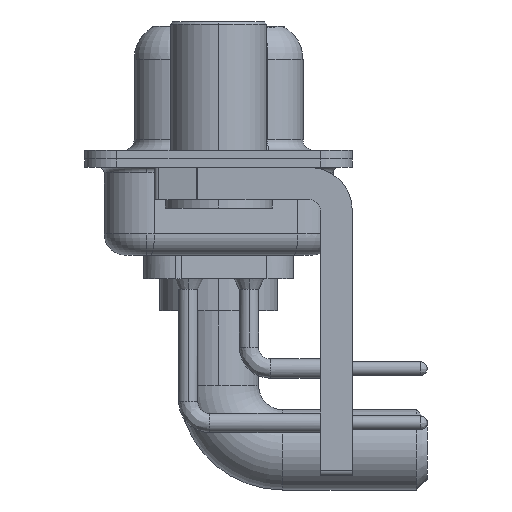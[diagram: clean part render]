
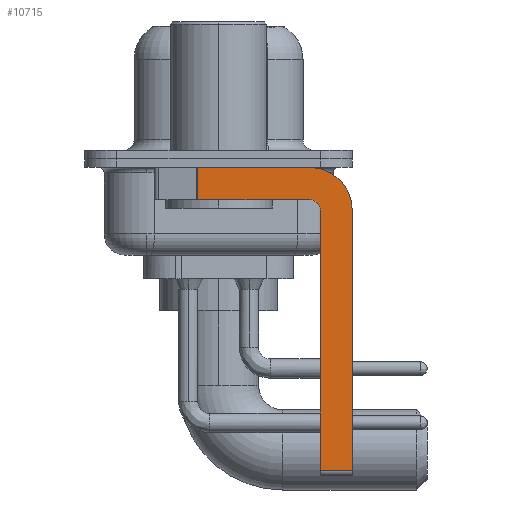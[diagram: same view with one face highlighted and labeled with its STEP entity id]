
A CAD part, left-side view. The second image highlights one B-rep face of the part: STEP entity #10715.
In plain terms, the highlighted planar face has unit normal (-1, 0, 0).
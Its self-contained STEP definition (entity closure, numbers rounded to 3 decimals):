
#270 = CARTESIAN_POINT ( 'NONE',  ( -2.9, 0.978, -1.9 ) ) ;
#313 = VECTOR ( 'NONE', #9322, 1000. ) ;
#455 = CARTESIAN_POINT ( 'NONE',  ( -2.9, -4.25, -1.9 ) ) ;
#612 = LINE ( 'NONE', #16915, #10787 ) ;
#702 = DIRECTION ( 'NONE',  ( 0., 0., -1. ) ) ;
#1063 = EDGE_CURVE ( 'NONE', #9135, #16388, #6700, .T. ) ;
#1362 = DIRECTION ( 'NONE',  ( -1., 0., 0. ) ) ;
#2097 = DIRECTION ( 'NONE',  ( 1., 0., 0. ) ) ;
#2965 = DIRECTION ( 'NONE',  ( 0., -1., 0. ) ) ;
#3438 = VERTEX_POINT ( 'NONE', #8987 ) ;
#4019 = VECTOR ( 'NONE', #702, 1000. ) ;
#4088 = VECTOR ( 'NONE', #7142, 1000. ) ;
#4329 = VECTOR ( 'NONE', #2965, 1000. ) ;
#4563 = DIRECTION ( 'NONE',  ( 0., 0., 1. ) ) ;
#4607 = CARTESIAN_POINT ( 'NONE',  ( -2.9, -4.75, -2.4 ) ) ;
#4699 = ORIENTED_EDGE ( 'NONE', *, *, #1063, .F. ) ;
#4745 = CIRCLE ( 'NONE', #13836, 0.5 ) ;
#5616 = PLANE ( 'NONE',  #11859 ) ;
#5619 = EDGE_CURVE ( 'NONE', #18272, #20762, #14762, .T. ) ;
#6700 = LINE ( 'NONE', #13361, #4088 ) ;
#7142 = DIRECTION ( 'NONE',  ( 0., 0., -1. ) ) ;
#7213 = FACE_OUTER_BOUND ( 'NONE', #13570, .T. ) ;
#7489 = DIRECTION ( 'NONE',  ( 0., -1., 0. ) ) ;
#7623 = CARTESIAN_POINT ( 'NONE',  ( -2.9, -4.25, -0.4 ) ) ;
#8331 = ORIENTED_EDGE ( 'NONE', *, *, #15761, .F. ) ;
#8383 = ORIENTED_EDGE ( 'NONE', *, *, #9776, .F. ) ;
#8558 = DIRECTION ( 'NONE',  ( 0., 0., -1. ) ) ;
#8987 = CARTESIAN_POINT ( 'NONE',  ( -2.9, -4.75, -14.55 ) ) ;
#9135 = VERTEX_POINT ( 'NONE', #17491 ) ;
#9322 = DIRECTION ( 'NONE',  ( 0., 0., 1. ) ) ;
#9467 = CIRCLE ( 'NONE', #19290, 2. ) ;
#9637 = EDGE_CURVE ( 'NONE', #14297, #12432, #4745, .T. ) ;
#9776 = EDGE_CURVE ( 'NONE', #14078, #9135, #9467, .T. ) ;
#10487 = CARTESIAN_POINT ( 'NONE',  ( -2.9, -4.25, -2.4 ) ) ;
#10715 = ADVANCED_FACE ( 'NONE', ( #7213 ), #5616, .F. ) ;
#10787 = VECTOR ( 'NONE', #19797, 1000. ) ;
#11312 = CARTESIAN_POINT ( 'NONE',  ( -2.9, -4.25, -14.55 ) ) ;
#11504 = LINE ( 'NONE', #19682, #313 ) ;
#11859 = AXIS2_PLACEMENT_3D ( 'NONE', #10487, #16946, #20717 ) ;
#12332 = LINE ( 'NONE', #18829, #18881 ) ;
#12432 = VERTEX_POINT ( 'NONE', #455 ) ;
#12444 = CARTESIAN_POINT ( 'NONE',  ( -2.9, 0.978, -1.9 ) ) ;
#13361 = CARTESIAN_POINT ( 'NONE',  ( -2.9, -6.25, -2.4 ) ) ;
#13570 = EDGE_LOOP ( 'NONE', ( #8331, #13980, #20934, #14658, #15207, #16603, #4699, #8383 ) ) ;
#13836 = AXIS2_PLACEMENT_3D ( 'NONE', #19074, #1362, #4563 ) ;
#13980 = ORIENTED_EDGE ( 'NONE', *, *, #5619, .T. ) ;
#14078 = VERTEX_POINT ( 'NONE', #7623 ) ;
#14297 = VERTEX_POINT ( 'NONE', #4607 ) ;
#14592 = LINE ( 'NONE', #11312, #4329 ) ;
#14658 = ORIENTED_EDGE ( 'NONE', *, *, #9637, .F. ) ;
#14762 = LINE ( 'NONE', #270, #4019 ) ;
#15207 = ORIENTED_EDGE ( 'NONE', *, *, #18730, .F. ) ;
#15461 = EDGE_CURVE ( 'NONE', #3438, #16388, #14592, .T. ) ;
#15761 = EDGE_CURVE ( 'NONE', #18272, #14078, #12332, .T. ) ;
#16388 = VERTEX_POINT ( 'NONE', #19127 ) ;
#16602 = CARTESIAN_POINT ( 'NONE',  ( -2.9, -4.25, -2.4 ) ) ;
#16603 = ORIENTED_EDGE ( 'NONE', *, *, #15461, .T. ) ;
#16643 = CARTESIAN_POINT ( 'NONE',  ( -2.9, 0.978, -0.4 ) ) ;
#16915 = CARTESIAN_POINT ( 'NONE',  ( -2.9, -4.25, -1.9 ) ) ;
#16946 = DIRECTION ( 'NONE',  ( 1., 0., 0. ) ) ;
#17044 = EDGE_CURVE ( 'NONE', #12432, #20762, #612, .T. ) ;
#17491 = CARTESIAN_POINT ( 'NONE',  ( -2.9, -6.25, -2.4 ) ) ;
#18272 = VERTEX_POINT ( 'NONE', #16643 ) ;
#18730 = EDGE_CURVE ( 'NONE', #3438, #14297, #11504, .T. ) ;
#18829 = CARTESIAN_POINT ( 'NONE',  ( -2.9, 3., -0.4 ) ) ;
#18881 = VECTOR ( 'NONE', #7489, 1000. ) ;
#19074 = CARTESIAN_POINT ( 'NONE',  ( -2.9, -4.25, -2.4 ) ) ;
#19127 = CARTESIAN_POINT ( 'NONE',  ( -2.9, -6.25, -14.55 ) ) ;
#19290 = AXIS2_PLACEMENT_3D ( 'NONE', #16602, #2097, #8558 ) ;
#19682 = CARTESIAN_POINT ( 'NONE',  ( -2.9, -4.75, -14.8 ) ) ;
#19797 = DIRECTION ( 'NONE',  ( 0., 1., 0. ) ) ;
#20717 = DIRECTION ( 'NONE',  ( 0., 0., -1. ) ) ;
#20762 = VERTEX_POINT ( 'NONE', #12444 ) ;
#20934 = ORIENTED_EDGE ( 'NONE', *, *, #17044, .F. ) ;
